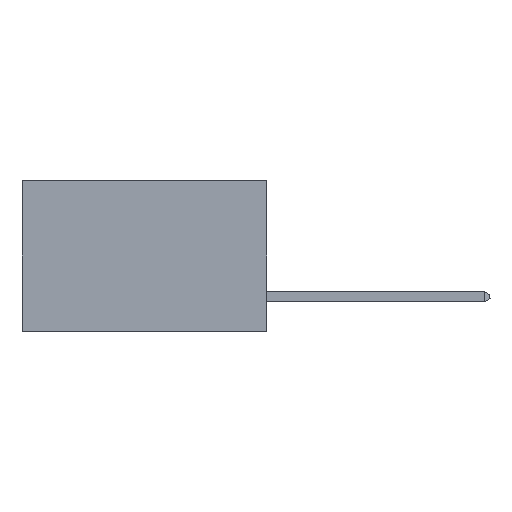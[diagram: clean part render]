
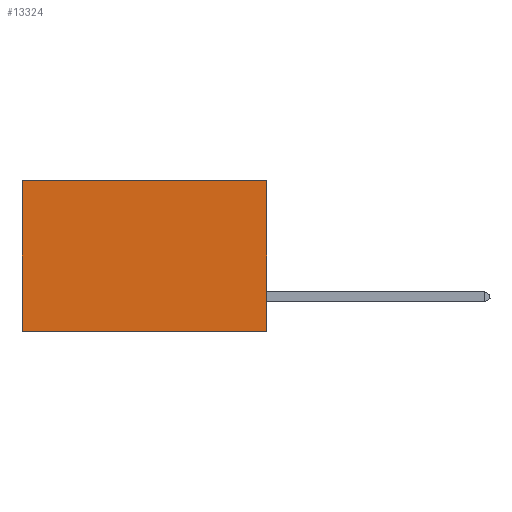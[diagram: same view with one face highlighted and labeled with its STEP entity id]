
A CAD part, left-side view. The second image highlights one B-rep face of the part: STEP entity #13324.
In plain terms, the highlighted planar face has unit normal (-1, 0, 0).
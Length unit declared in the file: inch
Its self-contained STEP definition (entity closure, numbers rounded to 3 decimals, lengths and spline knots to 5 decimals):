
#521 = CARTESIAN_POINT ( 'NONE',  ( 0.2875, 0., -0.37 ) ) ;
#1865 = DIRECTION ( 'NONE',  ( 0., 0., -1. ) ) ;
#2678 = FACE_OUTER_BOUND ( 'NONE', #32662, .T. ) ;
#4684 = ORIENTED_EDGE ( 'NONE', *, *, #5348, .T. ) ;
#4889 = DIRECTION ( 'NONE',  ( 0., 0., -1. ) ) ;
#5348 = EDGE_CURVE ( 'NONE', #10707, #13023, #23161, .T. ) ;
#6017 = CARTESIAN_POINT ( 'NONE',  ( 0.2875, 0.6, 0. ) ) ;
#6363 = ORIENTED_EDGE ( 'NONE', *, *, #10043, .F. ) ;
#8550 = EDGE_CURVE ( 'NONE', #22647, #13023, #16256, .T. ) ;
#8944 = CARTESIAN_POINT ( 'NONE',  ( 0.2875, 0., -0.37 ) ) ;
#9397 = DIRECTION ( 'NONE',  ( 0., 1., 0. ) ) ;
#10043 = EDGE_CURVE ( 'NONE', #19669, #22647, #30373, .T. ) ;
#10707 = VERTEX_POINT ( 'NONE', #6017 ) ;
#11096 = CARTESIAN_POINT ( 'NONE',  ( 0.2875, 0., 0. ) ) ;
#11595 = ORIENTED_EDGE ( 'NONE', *, *, #8550, .F. ) ;
#12848 = DIRECTION ( 'NONE',  ( 0., 1., 0. ) ) ;
#13023 = VERTEX_POINT ( 'NONE', #14530 ) ;
#13324 = ADVANCED_FACE ( 'NONE', ( #2678 ), #38636, .F. ) ;
#14530 = CARTESIAN_POINT ( 'NONE',  ( 0.2875, 0.6, -0.37 ) ) ;
#14961 = VECTOR ( 'NONE', #9397, 39.37008 ) ;
#15967 = CARTESIAN_POINT ( 'NONE',  ( 0.2875, 0.6, 0. ) ) ;
#16256 = LINE ( 'NONE', #521, #38642 ) ;
#16881 = AXIS2_PLACEMENT_3D ( 'NONE', #23221, #32328, #4889 ) ;
#18272 = LINE ( 'NONE', #18463, #14961 ) ;
#18463 = CARTESIAN_POINT ( 'NONE',  ( 0.2875, 0., 0. ) ) ;
#19669 = VERTEX_POINT ( 'NONE', #32825 ) ;
#22647 = VERTEX_POINT ( 'NONE', #8944 ) ;
#23161 = LINE ( 'NONE', #15967, #30251 ) ;
#23221 = CARTESIAN_POINT ( 'NONE',  ( 0.2875, 0., 0. ) ) ;
#25105 = EDGE_CURVE ( 'NONE', #19669, #10707, #18272, .T. ) ;
#25640 = VECTOR ( 'NONE', #1865, 39.37008 ) ;
#30251 = VECTOR ( 'NONE', #34528, 39.37008 ) ;
#30373 = LINE ( 'NONE', #11096, #25640 ) ;
#31569 = ORIENTED_EDGE ( 'NONE', *, *, #25105, .T. ) ;
#32328 = DIRECTION ( 'NONE',  ( 1., 0., 0. ) ) ;
#32662 = EDGE_LOOP ( 'NONE', ( #4684, #11595, #6363, #31569 ) ) ;
#32825 = CARTESIAN_POINT ( 'NONE',  ( 0.2875, 0., 0. ) ) ;
#34528 = DIRECTION ( 'NONE',  ( 0., 0., -1. ) ) ;
#38636 = PLANE ( 'NONE',  #16881 ) ;
#38642 = VECTOR ( 'NONE', #12848, 39.37008 ) ;
